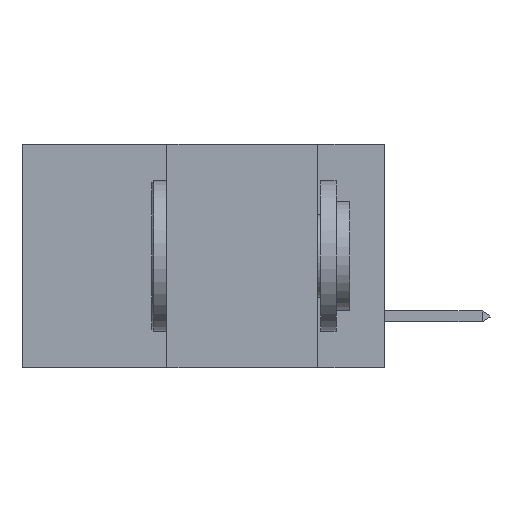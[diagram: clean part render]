
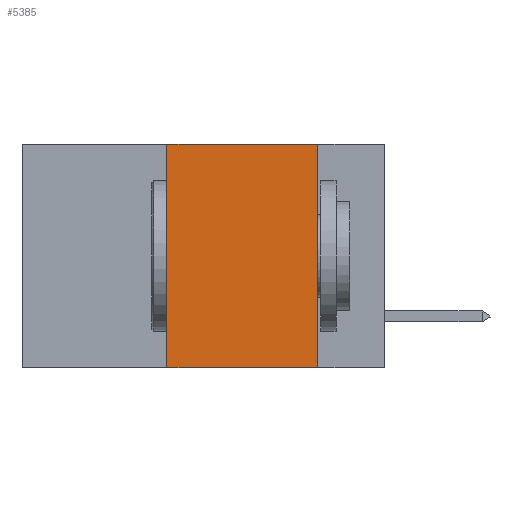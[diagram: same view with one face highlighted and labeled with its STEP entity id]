
A CAD part, left-side view. The second image highlights one B-rep face of the part: STEP entity #5385.
In plain terms, the highlighted planar face has unit normal (-1, 0, 0).
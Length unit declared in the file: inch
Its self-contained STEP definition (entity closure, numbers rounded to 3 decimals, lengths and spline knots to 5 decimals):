
#1389 = DIRECTION ( 'NONE',  ( 0., 0., -1. ) ) ;
#2068 = CARTESIAN_POINT ( 'NONE',  ( 0., 0.36, -0.37 ) ) ;
#3137 = EDGE_CURVE ( 'NONE', #24885, #12901, #24922, .T. ) ;
#3756 = LINE ( 'NONE', #10856, #20836 ) ;
#5385 = ADVANCED_FACE ( 'NONE', ( #12520 ), #18124, .F. ) ;
#5765 = CARTESIAN_POINT ( 'NONE',  ( 0., 0.11, -0.37 ) ) ;
#5965 = ORIENTED_EDGE ( 'NONE', *, *, #3137, .F. ) ;
#6135 = CARTESIAN_POINT ( 'NONE',  ( 0., 0.6, -0.37 ) ) ;
#6567 = CARTESIAN_POINT ( 'NONE',  ( 0., 0.6, 0. ) ) ;
#6856 = LINE ( 'NONE', #6135, #25299 ) ;
#7345 = ORIENTED_EDGE ( 'NONE', *, *, #18359, .F. ) ;
#7924 = VECTOR ( 'NONE', #23655, 39.37008 ) ;
#8678 = EDGE_CURVE ( 'NONE', #23911, #24885, #19407, .T. ) ;
#10713 = CARTESIAN_POINT ( 'NONE',  ( 0., 0.11, 0. ) ) ;
#10793 = EDGE_LOOP ( 'NONE', ( #7345, #5965, #25398, #23824 ) ) ;
#10856 = CARTESIAN_POINT ( 'NONE',  ( 0., 0.11, 0. ) ) ;
#12520 = FACE_OUTER_BOUND ( 'NONE', #10793, .T. ) ;
#12901 = VERTEX_POINT ( 'NONE', #10713 ) ;
#15543 = VERTEX_POINT ( 'NONE', #5765 ) ;
#16440 = CARTESIAN_POINT ( 'NONE',  ( 0., 0.36, 0. ) ) ;
#18124 = PLANE ( 'NONE',  #23187 ) ;
#18359 = EDGE_CURVE ( 'NONE', #12901, #15543, #3756, .T. ) ;
#18864 = DIRECTION ( 'NONE',  ( 0., 0., 1. ) ) ;
#19407 = LINE ( 'NONE', #16440, #27701 ) ;
#20676 = DIRECTION ( 'NONE',  ( 0., 0., -1. ) ) ;
#20836 = VECTOR ( 'NONE', #1389, 39.37008 ) ;
#21362 = CARTESIAN_POINT ( 'NONE',  ( 0., 0.6, 0. ) ) ;
#22016 = EDGE_CURVE ( 'NONE', #23911, #15543, #6856, .T. ) ;
#22800 = DIRECTION ( 'NONE',  ( 1., 0., 0. ) ) ;
#23187 = AXIS2_PLACEMENT_3D ( 'NONE', #6567, #22800, #20676 ) ;
#23655 = DIRECTION ( 'NONE',  ( 0., -1., 0. ) ) ;
#23824 = ORIENTED_EDGE ( 'NONE', *, *, #22016, .T. ) ;
#23911 = VERTEX_POINT ( 'NONE', #2068 ) ;
#24531 = DIRECTION ( 'NONE',  ( 0., -1., 0. ) ) ;
#24885 = VERTEX_POINT ( 'NONE', #27800 ) ;
#24922 = LINE ( 'NONE', #21362, #7924 ) ;
#25299 = VECTOR ( 'NONE', #24531, 39.37008 ) ;
#25398 = ORIENTED_EDGE ( 'NONE', *, *, #8678, .F. ) ;
#27701 = VECTOR ( 'NONE', #18864, 39.37008 ) ;
#27800 = CARTESIAN_POINT ( 'NONE',  ( 0., 0.36, 0. ) ) ;
